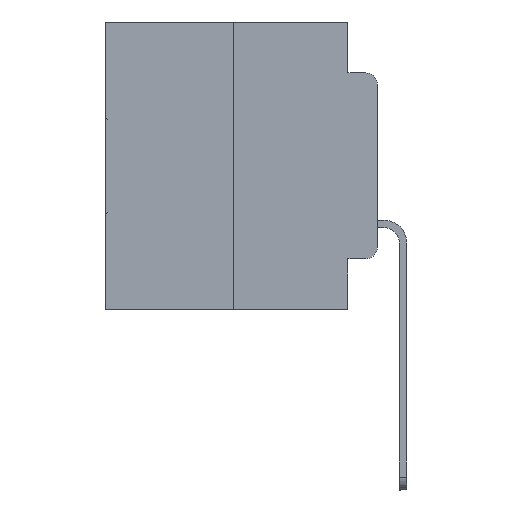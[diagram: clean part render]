
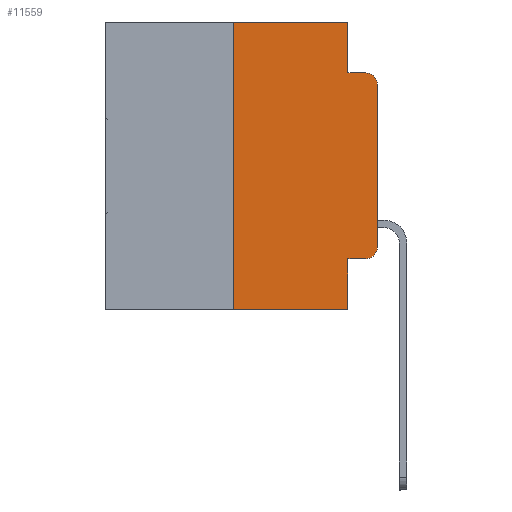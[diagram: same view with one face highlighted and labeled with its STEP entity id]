
A CAD part, left-side view. The second image highlights one B-rep face of the part: STEP entity #11559.
In plain terms, the highlighted planar face has unit normal (-1, 0, 0).
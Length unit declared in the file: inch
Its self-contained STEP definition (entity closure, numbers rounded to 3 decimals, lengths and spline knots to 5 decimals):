
#190 = EDGE_CURVE ( 'NONE', #907, #16279, #28160, .T. ) ;
#266 = CIRCLE ( 'NONE', #27991, 0.02 ) ;
#550 = ORIENTED_EDGE ( 'NONE', *, *, #1782, .F. ) ;
#907 = VERTEX_POINT ( 'NONE', #3056 ) ;
#917 = CARTESIAN_POINT ( 'NONE',  ( 0., 0.051, -0.0885 ) ) ;
#1321 = ORIENTED_EDGE ( 'NONE', *, *, #19826, .F. ) ;
#1782 = EDGE_CURVE ( 'NONE', #30809, #9828, #16522, .T. ) ;
#2118 = DIRECTION ( 'NONE',  ( 0., -1., 0. ) ) ;
#2436 = ORIENTED_EDGE ( 'NONE', *, *, #8376, .T. ) ;
#2504 = VECTOR ( 'NONE', #2118, 39.37008 ) ;
#2629 = CARTESIAN_POINT ( 'NONE',  ( 0., 0.051, -0.0885 ) ) ;
#2642 = FACE_OUTER_BOUND ( 'NONE', #31624, .T. ) ;
#2978 = AXIS2_PLACEMENT_3D ( 'NONE', #26496, #12061, #28914 ) ;
#3056 = CARTESIAN_POINT ( 'NONE',  ( 0., 0., -0.3915 ) ) ;
#3101 = EDGE_CURVE ( 'NONE', #28765, #20131, #22492, .T. ) ;
#3464 = ORIENTED_EDGE ( 'NONE', *, *, #190, .T. ) ;
#4312 = ORIENTED_EDGE ( 'NONE', *, *, #26869, .T. ) ;
#4684 = CARTESIAN_POINT ( 'NONE',  ( 0., 0.473, 0. ) ) ;
#5070 = EDGE_CURVE ( 'NONE', #9828, #17313, #27994, .T. ) ;
#5509 = ORIENTED_EDGE ( 'NONE', *, *, #29459, .F. ) ;
#6971 = VERTEX_POINT ( 'NONE', #20471 ) ;
#7253 = DIRECTION ( 'NONE',  ( 0., 0., -1. ) ) ;
#7437 = CARTESIAN_POINT ( 'NONE',  ( 0., 0.051, 0. ) ) ;
#7494 = ORIENTED_EDGE ( 'NONE', *, *, #3101, .T. ) ;
#7516 = CARTESIAN_POINT ( 'NONE',  ( 0., 0.473, 0. ) ) ;
#7668 = CARTESIAN_POINT ( 'NONE',  ( 0., 0.02, -0.1085 ) ) ;
#7820 = ORIENTED_EDGE ( 'NONE', *, *, #11531, .T. ) ;
#8003 = VECTOR ( 'NONE', #26346, 39.37008 ) ;
#8376 = EDGE_CURVE ( 'NONE', #16586, #18301, #22086, .T. ) ;
#8480 = VECTOR ( 'NONE', #30866, 39.37008 ) ;
#8959 = VECTOR ( 'NONE', #14392, 39.37008 ) ;
#9491 = CIRCLE ( 'NONE', #2978, 0.02 ) ;
#9828 = VERTEX_POINT ( 'NONE', #26352 ) ;
#9943 = DIRECTION ( 'NONE',  ( 0., 0., -1. ) ) ;
#10019 = DIRECTION ( 'NONE',  ( 0., 0., 1. ) ) ;
#10047 = VECTOR ( 'NONE', #10019, 39.37008 ) ;
#10074 = CARTESIAN_POINT ( 'NONE',  ( 0., 0.25, 0. ) ) ;
#10166 = DIRECTION ( 'NONE',  ( 0., 0., -1. ) ) ;
#11531 = EDGE_CURVE ( 'NONE', #20131, #907, #9491, .T. ) ;
#11559 = ADVANCED_FACE ( 'NONE', ( #2642 ), #19368, .F. ) ;
#11645 = CARTESIAN_POINT ( 'NONE',  ( 0., 0.473, -0.5 ) ) ;
#12061 = DIRECTION ( 'NONE',  ( -1., 0., 0. ) ) ;
#12170 = LINE ( 'NONE', #7437, #24279 ) ;
#12318 = DIRECTION ( 'NONE',  ( 0., -1., 0. ) ) ;
#13027 = AXIS2_PLACEMENT_3D ( 'NONE', #4684, #21790, #7253 ) ;
#13443 = CARTESIAN_POINT ( 'NONE',  ( 0., 0.02, -0.4115 ) ) ;
#14392 = DIRECTION ( 'NONE',  ( 0., 0., 1. ) ) ;
#14538 = VECTOR ( 'NONE', #12318, 39.37008 ) ;
#16232 = ORIENTED_EDGE ( 'NONE', *, *, #5070, .F. ) ;
#16279 = VERTEX_POINT ( 'NONE', #30977 ) ;
#16429 = LINE ( 'NONE', #19622, #10047 ) ;
#16522 = LINE ( 'NONE', #7516, #2504 ) ;
#16586 = VERTEX_POINT ( 'NONE', #23872 ) ;
#16907 = CARTESIAN_POINT ( 'NONE',  ( 0., 0., 0. ) ) ;
#17313 = VERTEX_POINT ( 'NONE', #2629 ) ;
#18301 = VERTEX_POINT ( 'NONE', #20853 ) ;
#18494 = DIRECTION ( 'NONE',  ( 0., -1., 0. ) ) ;
#19368 = PLANE ( 'NONE',  #13027 ) ;
#19541 = CARTESIAN_POINT ( 'NONE',  ( 0., 0.051, -0.4115 ) ) ;
#19622 = CARTESIAN_POINT ( 'NONE',  ( 0., 0.25, 0. ) ) ;
#19826 = EDGE_CURVE ( 'NONE', #16586, #30809, #16429, .T. ) ;
#20131 = VERTEX_POINT ( 'NONE', #13443 ) ;
#20471 = CARTESIAN_POINT ( 'NONE',  ( 0., 0.02, -0.0885 ) ) ;
#20853 = CARTESIAN_POINT ( 'NONE',  ( 0., 0.051, -0.5 ) ) ;
#21790 = DIRECTION ( 'NONE',  ( 1., 0., 0. ) ) ;
#22086 = LINE ( 'NONE', #11645, #8480 ) ;
#22492 = LINE ( 'NONE', #26559, #14538 ) ;
#23872 = CARTESIAN_POINT ( 'NONE',  ( 0., 0.25, -0.5 ) ) ;
#24279 = VECTOR ( 'NONE', #9943, 39.37008 ) ;
#24609 = DIRECTION ( 'NONE',  ( -1., 0., 0. ) ) ;
#24753 = VECTOR ( 'NONE', #18494, 39.37008 ) ;
#25310 = ORIENTED_EDGE ( 'NONE', *, *, #28460, .F. ) ;
#26346 = DIRECTION ( 'NONE',  ( 0., 0., -1. ) ) ;
#26352 = CARTESIAN_POINT ( 'NONE',  ( 0., 0.051, 0. ) ) ;
#26496 = CARTESIAN_POINT ( 'NONE',  ( 0., 0.02, -0.3915 ) ) ;
#26559 = CARTESIAN_POINT ( 'NONE',  ( 0., 0.051, -0.4115 ) ) ;
#26869 = EDGE_CURVE ( 'NONE', #16279, #6971, #266, .T. ) ;
#27991 = AXIS2_PLACEMENT_3D ( 'NONE', #7668, #24609, #10166 ) ;
#27994 = LINE ( 'NONE', #31020, #8003 ) ;
#28160 = LINE ( 'NONE', #16907, #8959 ) ;
#28460 = EDGE_CURVE ( 'NONE', #17313, #6971, #31073, .T. ) ;
#28765 = VERTEX_POINT ( 'NONE', #19541 ) ;
#28914 = DIRECTION ( 'NONE',  ( 0., 0., -1. ) ) ;
#29459 = EDGE_CURVE ( 'NONE', #28765, #18301, #12170, .T. ) ;
#30809 = VERTEX_POINT ( 'NONE', #10074 ) ;
#30866 = DIRECTION ( 'NONE',  ( 0., -1., 0. ) ) ;
#30977 = CARTESIAN_POINT ( 'NONE',  ( 0., 0., -0.1085 ) ) ;
#31020 = CARTESIAN_POINT ( 'NONE',  ( 0., 0.051, 0. ) ) ;
#31073 = LINE ( 'NONE', #917, #24753 ) ;
#31624 = EDGE_LOOP ( 'NONE', ( #3464, #4312, #25310, #16232, #550, #1321, #2436, #5509, #7494, #7820 ) ) ;
